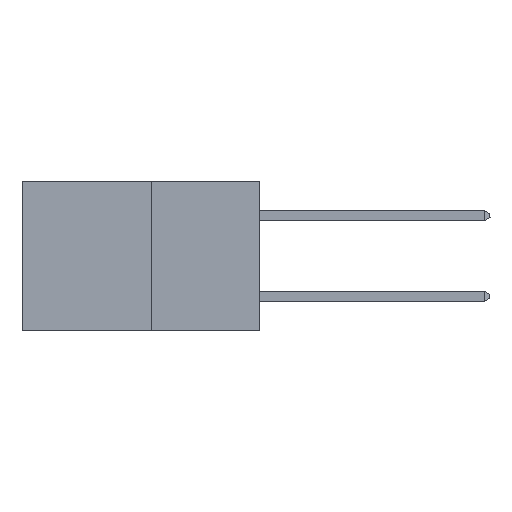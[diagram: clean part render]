
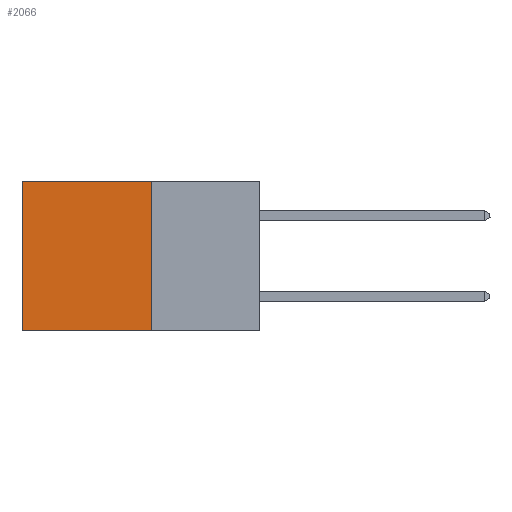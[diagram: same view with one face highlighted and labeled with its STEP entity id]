
A CAD part, left-side view. The second image highlights one B-rep face of the part: STEP entity #2066.
In plain terms, the highlighted planar face has unit normal (-1, 0, 0).
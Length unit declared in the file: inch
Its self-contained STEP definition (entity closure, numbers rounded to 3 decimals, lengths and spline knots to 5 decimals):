
#241 = VECTOR ( 'NONE', #9466, 39.37008 ) ;
#411 = VECTOR ( 'NONE', #1615, 39.37008 ) ;
#620 = EDGE_CURVE ( 'NONE', #837, #7775, #15522, .T. ) ;
#837 = VERTEX_POINT ( 'NONE', #2216 ) ;
#1051 = LINE ( 'NONE', #2266, #4170 ) ;
#1142 = DIRECTION ( 'NONE',  ( 0., 0., -1. ) ) ;
#1221 = CARTESIAN_POINT ( 'NONE',  ( 0.277, 0.59, -0.37 ) ) ;
#1615 = DIRECTION ( 'NONE',  ( 0., 0., -1. ) ) ;
#1699 = DIRECTION ( 'NONE',  ( 1., 0., 0. ) ) ;
#1717 = PLANE ( 'NONE',  #13357 ) ;
#1998 = ORIENTED_EDGE ( 'NONE', *, *, #11002, .F. ) ;
#2066 = ADVANCED_FACE ( 'NONE', ( #4417 ), #1717, .F. ) ;
#2092 = CARTESIAN_POINT ( 'NONE',  ( 0.277, 0.27, -0.37 ) ) ;
#2148 = VECTOR ( 'NONE', #14609, 39.37008 ) ;
#2216 = CARTESIAN_POINT ( 'NONE',  ( 0.277, 0.59, 0. ) ) ;
#2266 = CARTESIAN_POINT ( 'NONE',  ( 0.277, 0.27, -0.37 ) ) ;
#3374 = VERTEX_POINT ( 'NONE', #11024 ) ;
#3488 = EDGE_LOOP ( 'NONE', ( #16291, #1998, #16490, #12945 ) ) ;
#4170 = VECTOR ( 'NONE', #6269, 39.37008 ) ;
#4417 = FACE_OUTER_BOUND ( 'NONE', #3488, .T. ) ;
#5183 = VERTEX_POINT ( 'NONE', #11827 ) ;
#6269 = DIRECTION ( 'NONE',  ( 0., 1., 0. ) ) ;
#6839 = LINE ( 'NONE', #8126, #241 ) ;
#6854 = CARTESIAN_POINT ( 'NONE',  ( 0.277, 0.27, -0.37 ) ) ;
#7775 = VERTEX_POINT ( 'NONE', #1221 ) ;
#8126 = CARTESIAN_POINT ( 'NONE',  ( 0.277, 0.27, 0. ) ) ;
#9466 = DIRECTION ( 'NONE',  ( 0., 1., 0. ) ) ;
#10578 = EDGE_CURVE ( 'NONE', #3374, #837, #6839, .T. ) ;
#10866 = LINE ( 'NONE', #6854, #411 ) ;
#11002 = EDGE_CURVE ( 'NONE', #5183, #7775, #1051, .T. ) ;
#11024 = CARTESIAN_POINT ( 'NONE',  ( 0.277, 0.27, 0. ) ) ;
#11827 = CARTESIAN_POINT ( 'NONE',  ( 0.277, 0.27, -0.37 ) ) ;
#12379 = EDGE_CURVE ( 'NONE', #3374, #5183, #10866, .T. ) ;
#12945 = ORIENTED_EDGE ( 'NONE', *, *, #10578, .T. ) ;
#13357 = AXIS2_PLACEMENT_3D ( 'NONE', #2092, #1699, #1142 ) ;
#14228 = CARTESIAN_POINT ( 'NONE',  ( 0.277, 0.59, -0.37 ) ) ;
#14609 = DIRECTION ( 'NONE',  ( 0., 0., -1. ) ) ;
#15522 = LINE ( 'NONE', #14228, #2148 ) ;
#16291 = ORIENTED_EDGE ( 'NONE', *, *, #620, .T. ) ;
#16490 = ORIENTED_EDGE ( 'NONE', *, *, #12379, .F. ) ;
